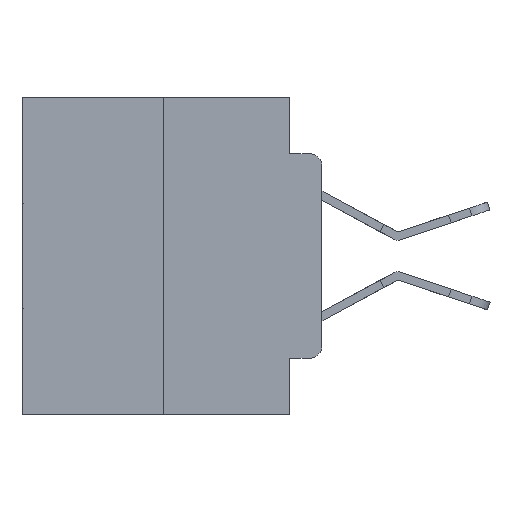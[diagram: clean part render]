
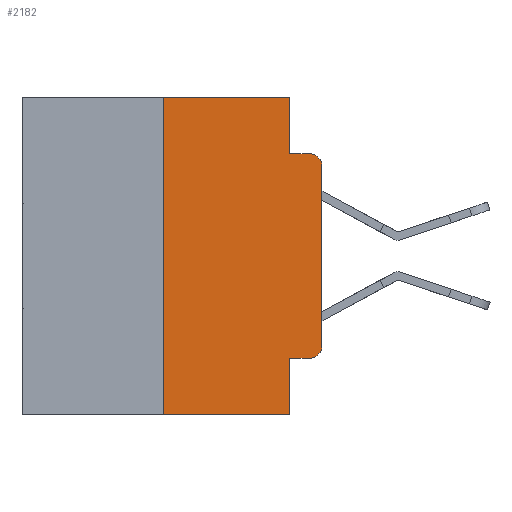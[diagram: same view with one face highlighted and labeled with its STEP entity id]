
A CAD part, left-side view. The second image highlights one B-rep face of the part: STEP entity #2182.
In plain terms, the highlighted planar face has unit normal (-1, 0, 0).
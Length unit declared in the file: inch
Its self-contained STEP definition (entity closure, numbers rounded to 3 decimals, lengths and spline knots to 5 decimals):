
#224 = EDGE_CURVE ( 'NONE', #20110, #1373, #25748, .T. ) ;
#234 = VECTOR ( 'NONE', #11445, 39.37008 ) ;
#543 = VECTOR ( 'NONE', #26788, 39.37008 ) ;
#751 = VERTEX_POINT ( 'NONE', #2923 ) ;
#1087 = CIRCLE ( 'NONE', #14134, 0.02 ) ;
#1282 = DIRECTION ( 'NONE',  ( 0., 0., 1. ) ) ;
#1373 = VERTEX_POINT ( 'NONE', #22847 ) ;
#1575 = EDGE_LOOP ( 'NONE', ( #15330, #22426, #5963, #8441, #19544, #19662, #15329, #25455, #15496, #27034 ) ) ;
#2182 = ADVANCED_FACE ( 'NONE', ( #28473 ), #21424, .F. ) ;
#2226 = CARTESIAN_POINT ( 'NONE',  ( 0., 0.051, 0. ) ) ;
#2232 = CARTESIAN_POINT ( 'NONE',  ( 0., 0.25, -0.5 ) ) ;
#2507 = VERTEX_POINT ( 'NONE', #18850 ) ;
#2923 = CARTESIAN_POINT ( 'NONE',  ( 0., 0.02, -0.4115 ) ) ;
#3838 = VECTOR ( 'NONE', #9069, 39.37008 ) ;
#4065 = DIRECTION ( 'NONE',  ( 0., 0., 1. ) ) ;
#4082 = CARTESIAN_POINT ( 'NONE',  ( 0., 0.473, -0.5 ) ) ;
#4148 = EDGE_CURVE ( 'NONE', #2507, #751, #13377, .T. ) ;
#4558 = LINE ( 'NONE', #5140, #26218 ) ;
#5140 = CARTESIAN_POINT ( 'NONE',  ( 0., 0.473, 0. ) ) ;
#5963 = ORIENTED_EDGE ( 'NONE', *, *, #224, .F. ) ;
#6588 = EDGE_CURVE ( 'NONE', #28327, #12906, #17211, .T. ) ;
#6629 = CARTESIAN_POINT ( 'NONE',  ( 0., 0.051, -0.4115 ) ) ;
#7580 = DIRECTION ( 'NONE',  ( 0., 0., -1. ) ) ;
#7879 = DIRECTION ( 'NONE',  ( 0., -1., 0. ) ) ;
#8441 = ORIENTED_EDGE ( 'NONE', *, *, #22751, .F. ) ;
#9069 = DIRECTION ( 'NONE',  ( 0., 0., -1. ) ) ;
#9274 = VERTEX_POINT ( 'NONE', #29799 ) ;
#9423 = CARTESIAN_POINT ( 'NONE',  ( 0., 0.02, -0.1085 ) ) ;
#11445 = DIRECTION ( 'NONE',  ( 0., -1., 0. ) ) ;
#12230 = AXIS2_PLACEMENT_3D ( 'NONE', #28183, #16463, #7580 ) ;
#12906 = VERTEX_POINT ( 'NONE', #23839 ) ;
#13294 = CARTESIAN_POINT ( 'NONE',  ( 0., 0.051, 0. ) ) ;
#13377 = LINE ( 'NONE', #6629, #25338 ) ;
#14134 = AXIS2_PLACEMENT_3D ( 'NONE', #29166, #20176, #24457 ) ;
#15080 = CARTESIAN_POINT ( 'NONE',  ( 0., 0., 0. ) ) ;
#15329 = ORIENTED_EDGE ( 'NONE', *, *, #6588, .T. ) ;
#15330 = ORIENTED_EDGE ( 'NONE', *, *, #29112, .T. ) ;
#15496 = ORIENTED_EDGE ( 'NONE', *, *, #4148, .T. ) ;
#16463 = DIRECTION ( 'NONE',  ( 1., 0., 0. ) ) ;
#16871 = EDGE_CURVE ( 'NONE', #2507, #12906, #22625, .T. ) ;
#17059 = VECTOR ( 'NONE', #7879, 39.37008 ) ;
#17211 = LINE ( 'NONE', #4082, #234 ) ;
#17379 = VERTEX_POINT ( 'NONE', #13294 ) ;
#17680 = CARTESIAN_POINT ( 'NONE',  ( 0., 0.25, 0. ) ) ;
#18428 = EDGE_CURVE ( 'NONE', #28327, #27970, #26849, .T. ) ;
#18850 = CARTESIAN_POINT ( 'NONE',  ( 0., 0.051, -0.4115 ) ) ;
#19544 = ORIENTED_EDGE ( 'NONE', *, *, #22834, .F. ) ;
#19662 = ORIENTED_EDGE ( 'NONE', *, *, #18428, .F. ) ;
#20110 = VERTEX_POINT ( 'NONE', #26086 ) ;
#20176 = DIRECTION ( 'NONE',  ( -1., 0., 0. ) ) ;
#20483 = EDGE_CURVE ( 'NONE', #751, #9274, #1087, .T. ) ;
#20705 = VECTOR ( 'NONE', #4065, 39.37008 ) ;
#21424 = PLANE ( 'NONE',  #12230 ) ;
#21730 = CARTESIAN_POINT ( 'NONE',  ( 0., 0.051, -0.0885 ) ) ;
#21970 = CARTESIAN_POINT ( 'NONE',  ( 0., 0.051, 0. ) ) ;
#22252 = CARTESIAN_POINT ( 'NONE',  ( 0., 0.25, 0. ) ) ;
#22426 = ORIENTED_EDGE ( 'NONE', *, *, #24801, .T. ) ;
#22625 = LINE ( 'NONE', #21970, #543 ) ;
#22735 = LINE ( 'NONE', #15080, #25618 ) ;
#22751 = EDGE_CURVE ( 'NONE', #17379, #20110, #29113, .T. ) ;
#22813 = DIRECTION ( 'NONE',  ( 0., -1., 0. ) ) ;
#22834 = EDGE_CURVE ( 'NONE', #27970, #17379, #4558, .T. ) ;
#22847 = CARTESIAN_POINT ( 'NONE',  ( 0., 0.02, -0.0885 ) ) ;
#23335 = CIRCLE ( 'NONE', #28330, 0.02 ) ;
#23624 = DIRECTION ( 'NONE',  ( 0., -1., 0. ) ) ;
#23839 = CARTESIAN_POINT ( 'NONE',  ( 0., 0.051, -0.5 ) ) ;
#24457 = DIRECTION ( 'NONE',  ( 0., 0., -1. ) ) ;
#24801 = EDGE_CURVE ( 'NONE', #27641, #1373, #23335, .T. ) ;
#25189 = CARTESIAN_POINT ( 'NONE',  ( 0., 0., -0.1085 ) ) ;
#25338 = VECTOR ( 'NONE', #22813, 39.37008 ) ;
#25455 = ORIENTED_EDGE ( 'NONE', *, *, #16871, .F. ) ;
#25590 = DIRECTION ( 'NONE',  ( 0., 0., -1. ) ) ;
#25618 = VECTOR ( 'NONE', #1282, 39.37008 ) ;
#25748 = LINE ( 'NONE', #21730, #17059 ) ;
#25893 = DIRECTION ( 'NONE',  ( -1., 0., 0. ) ) ;
#26086 = CARTESIAN_POINT ( 'NONE',  ( 0., 0.051, -0.0885 ) ) ;
#26218 = VECTOR ( 'NONE', #23624, 39.37008 ) ;
#26788 = DIRECTION ( 'NONE',  ( 0., 0., -1. ) ) ;
#26849 = LINE ( 'NONE', #17680, #20705 ) ;
#27034 = ORIENTED_EDGE ( 'NONE', *, *, #20483, .T. ) ;
#27641 = VERTEX_POINT ( 'NONE', #25189 ) ;
#27970 = VERTEX_POINT ( 'NONE', #22252 ) ;
#28183 = CARTESIAN_POINT ( 'NONE',  ( 0., 0.473, 0. ) ) ;
#28327 = VERTEX_POINT ( 'NONE', #2232 ) ;
#28330 = AXIS2_PLACEMENT_3D ( 'NONE', #9423, #25893, #25590 ) ;
#28473 = FACE_OUTER_BOUND ( 'NONE', #1575, .T. ) ;
#29112 = EDGE_CURVE ( 'NONE', #9274, #27641, #22735, .T. ) ;
#29113 = LINE ( 'NONE', #2226, #3838 ) ;
#29166 = CARTESIAN_POINT ( 'NONE',  ( 0., 0.02, -0.3915 ) ) ;
#29799 = CARTESIAN_POINT ( 'NONE',  ( 0., 0., -0.3915 ) ) ;
